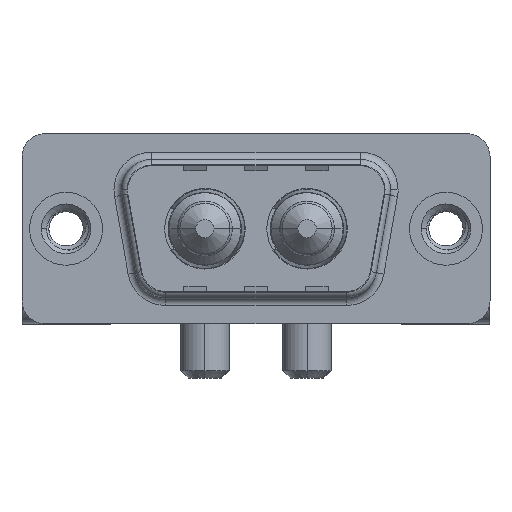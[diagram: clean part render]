
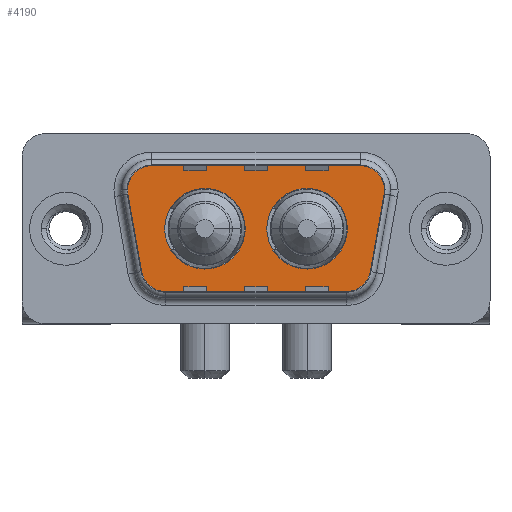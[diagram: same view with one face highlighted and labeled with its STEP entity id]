
A CAD part, top view. The second image highlights one B-rep face of the part: STEP entity #4190.
In plain terms, the highlighted planar face has unit normal (0, 0, 1).
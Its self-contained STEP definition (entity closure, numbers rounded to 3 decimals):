
#168 = AXIS2_PLACEMENT_3D ( 'NONE', #10279, #8344, #6294 ) ;
#295 = DIRECTION ( 'NONE',  ( 0., 0., 1. ) ) ;
#299 = DIRECTION ( 'NONE',  ( -1., 0., 0. ) ) ;
#325 = EDGE_CURVE ( 'NONE', #2453, #4519, #7573, .T. ) ;
#428 = DIRECTION ( 'NONE',  ( 0., 0., 1. ) ) ;
#439 = CARTESIAN_POINT ( 'NONE',  ( 5.436, 4.9, 0. ) ) ;
#781 = CARTESIAN_POINT ( 'NONE',  ( 21.534, 2.553, 0. ) ) ;
#783 = EDGE_CURVE ( 'NONE', #3274, #1813, #7797, .T. ) ;
#871 = ORIENTED_EDGE ( 'NONE', *, *, #5348, .T. ) ;
#901 = LINE ( 'NONE', #12297, #11828 ) ;
#909 = ORIENTED_EDGE ( 'NONE', *, *, #7439, .T. ) ;
#1023 = DIRECTION ( 'NONE',  ( 0.174, -0.985, 0. ) ) ;
#1050 = FACE_OUTER_BOUND ( 'NONE', #9098, .T. ) ;
#1182 = CARTESIAN_POINT ( 'NONE',  ( 19.564, 2.9, 0. ) ) ;
#1213 = ORIENTED_EDGE ( 'NONE', *, *, #783, .F. ) ;
#1335 = DIRECTION ( 'NONE',  ( 0., 0., 1. ) ) ;
#1487 = EDGE_CURVE ( 'NONE', #6555, #8981, #7480, .T. ) ;
#1576 = CIRCLE ( 'NONE', #168, 2.65 ) ;
#1813 = VERTEX_POINT ( 'NONE', #12087 ) ;
#1816 = CARTESIAN_POINT ( 'NONE',  ( 21.534, 2.553, 0. ) ) ;
#1822 = DIRECTION ( 'NONE',  ( 0., 0., 1. ) ) ;
#1982 = AXIS2_PLACEMENT_3D ( 'NONE', #5216, #11149, #3537 ) ;
#2119 = AXIS2_PLACEMENT_3D ( 'NONE', #10919, #11787, #6179 ) ;
#2319 = CARTESIAN_POINT ( 'NONE',  ( 19.564, 2.9, 0. ) ) ;
#2361 = LINE ( 'NONE', #4338, #11629 ) ;
#2453 = VERTEX_POINT ( 'NONE', #11971 ) ;
#2543 = ORIENTED_EDGE ( 'NONE', *, *, #7413, .F. ) ;
#2705 = ORIENTED_EDGE ( 'NONE', *, *, #11223, .T. ) ;
#2759 = CIRCLE ( 'NONE', #6398, 2. ) ;
#2772 = ORIENTED_EDGE ( 'NONE', *, *, #10464, .T. ) ;
#2924 = EDGE_CURVE ( 'NONE', #12002, #4697, #2361, .T. ) ;
#3274 = VERTEX_POINT ( 'NONE', #4084 ) ;
#3284 = ORIENTED_EDGE ( 'NONE', *, *, #325, .T. ) ;
#3398 = EDGE_CURVE ( 'NONE', #6082, #6600, #3668, .T. ) ;
#3537 = DIRECTION ( 'NONE',  ( -1., 0., 0. ) ) ;
#3668 = CIRCLE ( 'NONE', #9630, 2.65 ) ;
#3710 = VERTEX_POINT ( 'NONE', #6915 ) ;
#3776 = VERTEX_POINT ( 'NONE', #439 ) ;
#3955 = ORIENTED_EDGE ( 'NONE', *, *, #6794, .T. ) ;
#3957 = CIRCLE ( 'NONE', #1982, 2. ) ;
#3970 = PLANE ( 'NONE',  #6673 ) ;
#4084 = CARTESIAN_POINT ( 'NONE',  ( 11.79, 0., 0. ) ) ;
#4190 = ADVANCED_FACE ( 'NONE', ( #8834, #10525, #1050 ), #3970, .T. ) ;
#4200 = ORIENTED_EDGE ( 'NONE', *, *, #4810, .T. ) ;
#4276 = EDGE_LOOP ( 'NONE', ( #1213, #2543 ) ) ;
#4338 = CARTESIAN_POINT ( 'NONE',  ( 6.459, -4.9, 0. ) ) ;
#4412 = AXIS2_PLACEMENT_3D ( 'NONE', #9872, #1335, #11743 ) ;
#4519 = VERTEX_POINT ( 'NONE', #7724 ) ;
#4630 = DIRECTION ( 'NONE',  ( 1., 0., 0. ) ) ;
#4697 = VERTEX_POINT ( 'NONE', #11851 ) ;
#4717 = ORIENTED_EDGE ( 'NONE', *, *, #1487, .T. ) ;
#4810 = EDGE_CURVE ( 'NONE', #3776, #3710, #9464, .T. ) ;
#4815 = VECTOR ( 'NONE', #6605, 1000. ) ;
#4835 = CARTESIAN_POINT ( 'NONE',  ( 18.541, -2.9, 0. ) ) ;
#5216 = CARTESIAN_POINT ( 'NONE',  ( 6.459, -2.9, 0. ) ) ;
#5348 = EDGE_CURVE ( 'NONE', #4519, #3776, #11158, .T. ) ;
#5468 = AXIS2_PLACEMENT_3D ( 'NONE', #8200, #12004, #4630 ) ;
#5486 = CARTESIAN_POINT ( 'NONE',  ( 6.459, -4.9, 0. ) ) ;
#5738 = DIRECTION ( 'NONE',  ( 1., 0., 0. ) ) ;
#6076 = ORIENTED_EDGE ( 'NONE', *, *, #6416, .F. ) ;
#6082 = VERTEX_POINT ( 'NONE', #6610 ) ;
#6109 = DIRECTION ( 'NONE',  ( 0., 0., 1. ) ) ;
#6179 = DIRECTION ( 'NONE',  ( 1., 0., 0. ) ) ;
#6221 = DIRECTION ( 'NONE',  ( 1., 0., 0. ) ) ;
#6294 = DIRECTION ( 'NONE',  ( 1., 0., 0. ) ) ;
#6398 = AXIS2_PLACEMENT_3D ( 'NONE', #11441, #7746, #10441 ) ;
#6416 = EDGE_CURVE ( 'NONE', #6600, #6082, #1576, .T. ) ;
#6555 = VERTEX_POINT ( 'NONE', #11343 ) ;
#6600 = VERTEX_POINT ( 'NONE', #7523 ) ;
#6605 = DIRECTION ( 'NONE',  ( 0.174, 0.985, 0. ) ) ;
#6610 = CARTESIAN_POINT ( 'NONE',  ( 18.51, 0., 0. ) ) ;
#6673 = AXIS2_PLACEMENT_3D ( 'NONE', #4835, #295, #7773 ) ;
#6678 = CARTESIAN_POINT ( 'NONE',  ( 15.86, 0., 0. ) ) ;
#6747 = VERTEX_POINT ( 'NONE', #6901 ) ;
#6794 = EDGE_CURVE ( 'NONE', #6747, #12002, #3957, .T. ) ;
#6901 = CARTESIAN_POINT ( 'NONE',  ( 4.489, -3.247, 0. ) ) ;
#6915 = CARTESIAN_POINT ( 'NONE',  ( 3.466, 2.553, 0. ) ) ;
#7381 = AXIS2_PLACEMENT_3D ( 'NONE', #1182, #428, #299 ) ;
#7413 = EDGE_CURVE ( 'NONE', #1813, #3274, #10837, .T. ) ;
#7439 = EDGE_CURVE ( 'NONE', #3710, #6747, #901, .T. ) ;
#7480 = LINE ( 'NONE', #1816, #4815 ) ;
#7523 = CARTESIAN_POINT ( 'NONE',  ( 13.21, 0., 0. ) ) ;
#7573 = CIRCLE ( 'NONE', #7381, 2. ) ;
#7724 = CARTESIAN_POINT ( 'NONE',  ( 19.564, 4.9, 0. ) ) ;
#7746 = DIRECTION ( 'NONE',  ( 0., 0., 1. ) ) ;
#7773 = DIRECTION ( 'NONE',  ( 1., 0., 0. ) ) ;
#7797 = CIRCLE ( 'NONE', #4412, 2.65 ) ;
#7853 = DIRECTION ( 'NONE',  ( -1., 0., 0. ) ) ;
#8142 = CIRCLE ( 'NONE', #8348, 2. ) ;
#8200 = CARTESIAN_POINT ( 'NONE',  ( 9.14, 0., 0. ) ) ;
#8344 = DIRECTION ( 'NONE',  ( 0., 0., 1. ) ) ;
#8348 = AXIS2_PLACEMENT_3D ( 'NONE', #2319, #6109, #7853 ) ;
#8834 = FACE_BOUND ( 'NONE', #9048, .T. ) ;
#8981 = VERTEX_POINT ( 'NONE', #781 ) ;
#9048 = EDGE_LOOP ( 'NONE', ( #10619, #6076 ) ) ;
#9098 = EDGE_LOOP ( 'NONE', ( #2705, #4717, #2772, #3284, #871, #4200, #909, #3955, #12007 ) ) ;
#9160 = DIRECTION ( 'NONE',  ( -1., 0., 0. ) ) ;
#9464 = CIRCLE ( 'NONE', #2119, 2. ) ;
#9476 = VECTOR ( 'NONE', #9160, 1000. ) ;
#9630 = AXIS2_PLACEMENT_3D ( 'NONE', #6678, #1822, #5738 ) ;
#9872 = CARTESIAN_POINT ( 'NONE',  ( 9.14, 0., 0. ) ) ;
#10279 = CARTESIAN_POINT ( 'NONE',  ( 15.86, 0., 0. ) ) ;
#10441 = DIRECTION ( 'NONE',  ( 1., 0., 0. ) ) ;
#10464 = EDGE_CURVE ( 'NONE', #8981, #2453, #8142, .T. ) ;
#10525 = FACE_BOUND ( 'NONE', #4276, .T. ) ;
#10619 = ORIENTED_EDGE ( 'NONE', *, *, #3398, .F. ) ;
#10837 = CIRCLE ( 'NONE', #5468, 2.65 ) ;
#10919 = CARTESIAN_POINT ( 'NONE',  ( 5.436, 2.9, 0. ) ) ;
#11149 = DIRECTION ( 'NONE',  ( 0., 0., 1. ) ) ;
#11158 = LINE ( 'NONE', #11214, #9476 ) ;
#11214 = CARTESIAN_POINT ( 'NONE',  ( 5.436, 4.9, 0. ) ) ;
#11223 = EDGE_CURVE ( 'NONE', #4697, #6555, #2759, .T. ) ;
#11343 = CARTESIAN_POINT ( 'NONE',  ( 20.511, -3.247, 0. ) ) ;
#11441 = CARTESIAN_POINT ( 'NONE',  ( 18.541, -2.9, 0. ) ) ;
#11629 = VECTOR ( 'NONE', #6221, 1000. ) ;
#11743 = DIRECTION ( 'NONE',  ( 1., 0., 0. ) ) ;
#11787 = DIRECTION ( 'NONE',  ( 0., 0., 1. ) ) ;
#11828 = VECTOR ( 'NONE', #1023, 1000. ) ;
#11851 = CARTESIAN_POINT ( 'NONE',  ( 18.541, -4.9, 0. ) ) ;
#11971 = CARTESIAN_POINT ( 'NONE',  ( 21.564, 2.9, 0. ) ) ;
#12002 = VERTEX_POINT ( 'NONE', #5486 ) ;
#12004 = DIRECTION ( 'NONE',  ( 0., 0., 1. ) ) ;
#12007 = ORIENTED_EDGE ( 'NONE', *, *, #2924, .T. ) ;
#12087 = CARTESIAN_POINT ( 'NONE',  ( 6.49, 0., 0. ) ) ;
#12297 = CARTESIAN_POINT ( 'NONE',  ( 3.466, 2.553, 0. ) ) ;
